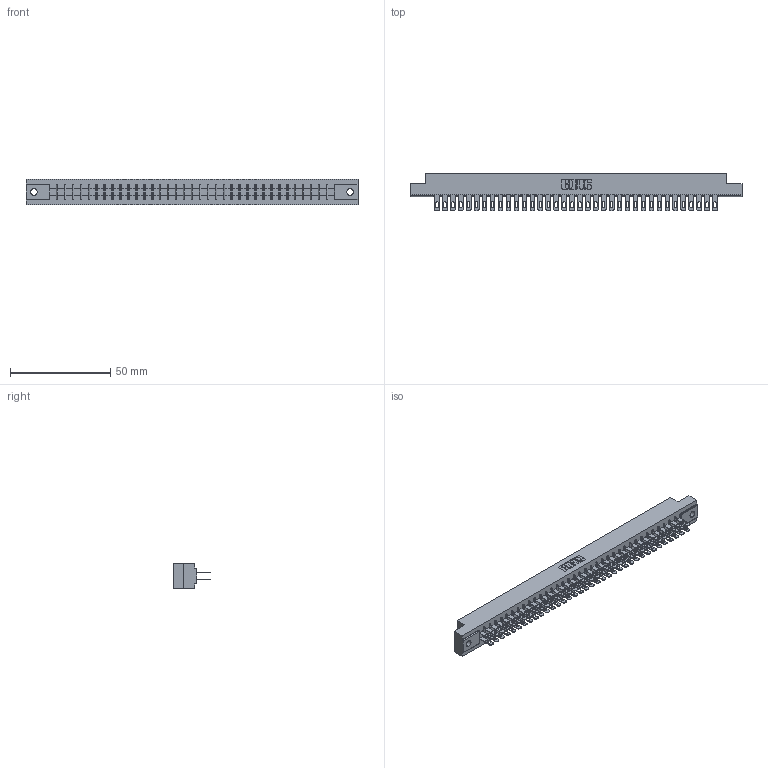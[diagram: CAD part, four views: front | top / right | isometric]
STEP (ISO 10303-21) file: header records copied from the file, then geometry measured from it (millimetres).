
FILE_DESCRIPTION (( 'STEP AP203' ), '1' );
FILE_NAME ('315-072-500-202.STEP', '2019-09-10T21:39:28', ( '' ), ( '' ), 'SwSTEP 2.0', 'SolidWorks 2016', '' );
FILE_SCHEMA (( 'CONFIG_CONTROL_DESIGN' ));
Length unit declared in the file: inch
Products named in the file (3): 315-072-500-202; 305-290-001_500; 305 Part_.128 Dia
Assembly tree (73 placements, depth 2):
  315-072-500-202
    305 Part_.128 Dia
    305-290-001_500  x72
Bounding box: 165.66 x 18.85 x 12.7 mm (x, y, z)
Volume: 17434.3 mm3; surface area: 23175.4 mm2
Topology: 73 solids, 73 shells, 3716 faces, 10648 edges, 6904 vertices
Faces by surface type: plane 2084, cylinder 1488, sphere 144
Entity records: 39733 total; most frequent: CARTESIAN_POINT 6574, ORIENTED_EDGE 6524, DIRECTION 6366, EDGE_CURVE 3262, VECTOR 2630, LINE 2630, VERTEX_POINT 2076, AXIS2_PLACEMENT_3D 1868
